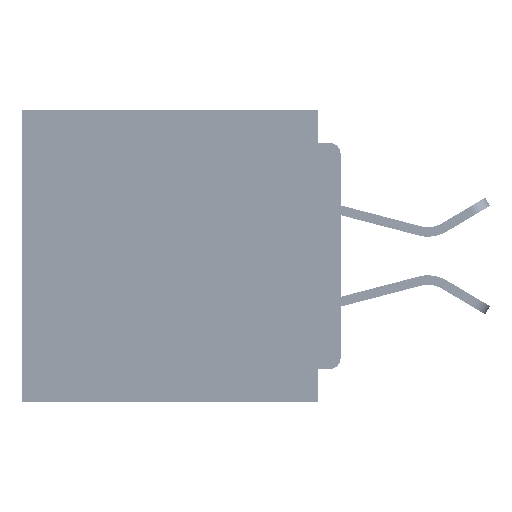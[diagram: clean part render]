
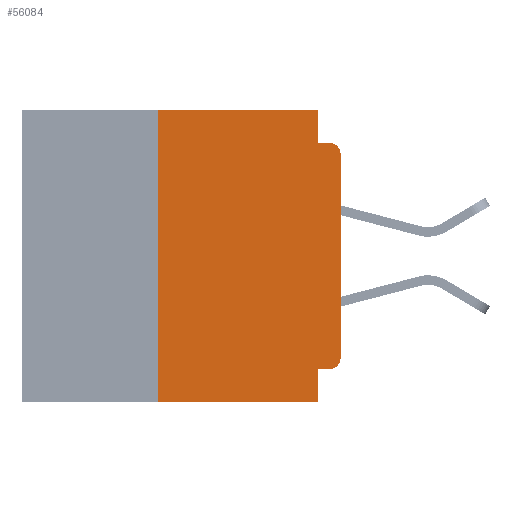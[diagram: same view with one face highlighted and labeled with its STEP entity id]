
A CAD part, left-side view. The second image highlights one B-rep face of the part: STEP entity #56084.
In plain terms, the highlighted planar face has unit normal (-1, 0, 0).
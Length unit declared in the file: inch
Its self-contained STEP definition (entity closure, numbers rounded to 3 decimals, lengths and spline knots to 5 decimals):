
#2589 = EDGE_LOOP ( 'NONE', ( #64266, #8690, #37856, #32117, #51288, #22043, #42055, #68194, #10691, #40504 ) ) ;
#4801 = CARTESIAN_POINT ( 'NONE',  ( 0., 0., -0.355 ) ) ;
#6203 = CARTESIAN_POINT ( 'NONE',  ( 0., 0.437, 0. ) ) ;
#6510 = VERTEX_POINT ( 'NONE', #24990 ) ;
#6711 = CARTESIAN_POINT ( 'NONE',  ( 0., 0., -0.06 ) ) ;
#8381 = EDGE_CURVE ( 'NONE', #54777, #41856, #13076, .T. ) ;
#8690 = ORIENTED_EDGE ( 'NONE', *, *, #25701, .T. ) ;
#9265 = VERTEX_POINT ( 'NONE', #13409 ) ;
#10038 = AXIS2_PLACEMENT_3D ( 'NONE', #26996, #42926, #11222 ) ;
#10363 = VECTOR ( 'NONE', #26342, 39.37008 ) ;
#10691 = ORIENTED_EDGE ( 'NONE', *, *, #8381, .F. ) ;
#11015 = CARTESIAN_POINT ( 'NONE',  ( 0., 0.015, -0.355 ) ) ;
#11222 = DIRECTION ( 'NONE',  ( 0., 0., -1. ) ) ;
#12171 = EDGE_CURVE ( 'NONE', #6510, #62787, #26862, .T. ) ;
#12248 = CARTESIAN_POINT ( 'NONE',  ( 0., 0.031, -0.045 ) ) ;
#13076 = LINE ( 'NONE', #4801, #37879 ) ;
#13409 = CARTESIAN_POINT ( 'NONE',  ( 0., 0., -0.34 ) ) ;
#13635 = FACE_OUTER_BOUND ( 'NONE', #2589, .T. ) ;
#13829 = CARTESIAN_POINT ( 'NONE',  ( 0., 0.015, -0.045 ) ) ;
#14337 = CARTESIAN_POINT ( 'NONE',  ( 0., 0.031, 0. ) ) ;
#15540 = DIRECTION ( 'NONE',  ( 0., 0., -1. ) ) ;
#16888 = VECTOR ( 'NONE', #21941, 39.37008 ) ;
#17500 = DIRECTION ( 'NONE',  ( 0., 0., -1. ) ) ;
#18627 = AXIS2_PLACEMENT_3D ( 'NONE', #24782, #61763, #30052 ) ;
#19261 = EDGE_CURVE ( 'NONE', #63543, #34029, #23483, .T. ) ;
#19560 = DIRECTION ( 'NONE',  ( 0., -1., 0. ) ) ;
#19850 = EDGE_CURVE ( 'NONE', #54777, #9265, #26784, .T. ) ;
#20635 = EDGE_CURVE ( 'NONE', #62787, #50531, #34911, .T. ) ;
#20881 = CARTESIAN_POINT ( 'NONE',  ( 0., 0.031, 0. ) ) ;
#21941 = DIRECTION ( 'NONE',  ( 0., 0., 1. ) ) ;
#22043 = ORIENTED_EDGE ( 'NONE', *, *, #28711, .F. ) ;
#23483 = LINE ( 'NONE', #56301, #49948 ) ;
#23570 = VECTOR ( 'NONE', #37915, 39.37008 ) ;
#24782 = CARTESIAN_POINT ( 'NONE',  ( 0., 0.015, -0.34 ) ) ;
#24990 = CARTESIAN_POINT ( 'NONE',  ( 0., 0.25, 0. ) ) ;
#25701 = EDGE_CURVE ( 'NONE', #37098, #55775, #38275, .T. ) ;
#26140 = LINE ( 'NONE', #67827, #10363 ) ;
#26342 = DIRECTION ( 'NONE',  ( 0., -1., 0. ) ) ;
#26784 = CIRCLE ( 'NONE', #18627, 0.015 ) ;
#26862 = LINE ( 'NONE', #6203, #23570 ) ;
#26996 = CARTESIAN_POINT ( 'NONE',  ( 0., 0.437, 0. ) ) ;
#28111 = CARTESIAN_POINT ( 'NONE',  ( 0., 0.031, -0.4 ) ) ;
#28552 = LINE ( 'NONE', #40647, #67467 ) ;
#28711 = EDGE_CURVE ( 'NONE', #63543, #6510, #45024, .T. ) ;
#30052 = DIRECTION ( 'NONE',  ( 0., 0., -1. ) ) ;
#31077 = DIRECTION ( 'NONE',  ( -1., 0., 0. ) ) ;
#31200 = DIRECTION ( 'NONE',  ( 0., 1., 0. ) ) ;
#32117 = ORIENTED_EDGE ( 'NONE', *, *, #20635, .F. ) ;
#34029 = VERTEX_POINT ( 'NONE', #65155 ) ;
#34911 = LINE ( 'NONE', #20881, #47362 ) ;
#37098 = VERTEX_POINT ( 'NONE', #6711 ) ;
#37856 = ORIENTED_EDGE ( 'NONE', *, *, #45483, .F. ) ;
#37879 = VECTOR ( 'NONE', #31200, 39.37008 ) ;
#37915 = DIRECTION ( 'NONE',  ( 0., -1., 0. ) ) ;
#38055 = CARTESIAN_POINT ( 'NONE',  ( 0., 0.25, -0.4 ) ) ;
#38275 = CIRCLE ( 'NONE', #46760, 0.015 ) ;
#40504 = ORIENTED_EDGE ( 'NONE', *, *, #19850, .T. ) ;
#40647 = CARTESIAN_POINT ( 'NONE',  ( 0., 0., 0. ) ) ;
#41856 = VERTEX_POINT ( 'NONE', #59905 ) ;
#42055 = ORIENTED_EDGE ( 'NONE', *, *, #19261, .T. ) ;
#42926 = DIRECTION ( 'NONE',  ( 1., 0., 0. ) ) ;
#45024 = LINE ( 'NONE', #38055, #16888 ) ;
#45483 = EDGE_CURVE ( 'NONE', #50531, #55775, #26140, .T. ) ;
#45895 = VECTOR ( 'NONE', #17500, 39.37008 ) ;
#45981 = DIRECTION ( 'NONE',  ( 0., 0., 1. ) ) ;
#46760 = AXIS2_PLACEMENT_3D ( 'NONE', #62773, #31077, #68087 ) ;
#47362 = VECTOR ( 'NONE', #15540, 39.37008 ) ;
#49948 = VECTOR ( 'NONE', #19560, 39.37008 ) ;
#50531 = VERTEX_POINT ( 'NONE', #12248 ) ;
#51288 = ORIENTED_EDGE ( 'NONE', *, *, #12171, .F. ) ;
#54777 = VERTEX_POINT ( 'NONE', #11015 ) ;
#55775 = VERTEX_POINT ( 'NONE', #13829 ) ;
#55827 = EDGE_CURVE ( 'NONE', #9265, #37098, #28552, .T. ) ;
#56084 = ADVANCED_FACE ( 'NONE', ( #13635 ), #58676, .F. ) ;
#56198 = EDGE_CURVE ( 'NONE', #41856, #34029, #59957, .T. ) ;
#56301 = CARTESIAN_POINT ( 'NONE',  ( 0., 0.437, -0.4 ) ) ;
#58676 = PLANE ( 'NONE',  #10038 ) ;
#59905 = CARTESIAN_POINT ( 'NONE',  ( 0., 0.031, -0.355 ) ) ;
#59957 = LINE ( 'NONE', #28111, #45895 ) ;
#61763 = DIRECTION ( 'NONE',  ( -1., 0., 0. ) ) ;
#62773 = CARTESIAN_POINT ( 'NONE',  ( 0., 0.015, -0.06 ) ) ;
#62787 = VERTEX_POINT ( 'NONE', #14337 ) ;
#63543 = VERTEX_POINT ( 'NONE', #68139 ) ;
#64266 = ORIENTED_EDGE ( 'NONE', *, *, #55827, .T. ) ;
#65155 = CARTESIAN_POINT ( 'NONE',  ( 0., 0.031, -0.4 ) ) ;
#67467 = VECTOR ( 'NONE', #45981, 39.37008 ) ;
#67827 = CARTESIAN_POINT ( 'NONE',  ( 0., 0., -0.045 ) ) ;
#68087 = DIRECTION ( 'NONE',  ( 0., 0., -1. ) ) ;
#68139 = CARTESIAN_POINT ( 'NONE',  ( 0., 0.25, -0.4 ) ) ;
#68194 = ORIENTED_EDGE ( 'NONE', *, *, #56198, .F. ) ;
